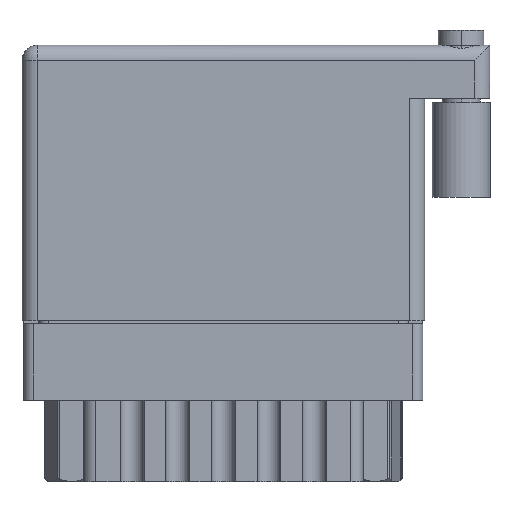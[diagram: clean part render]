
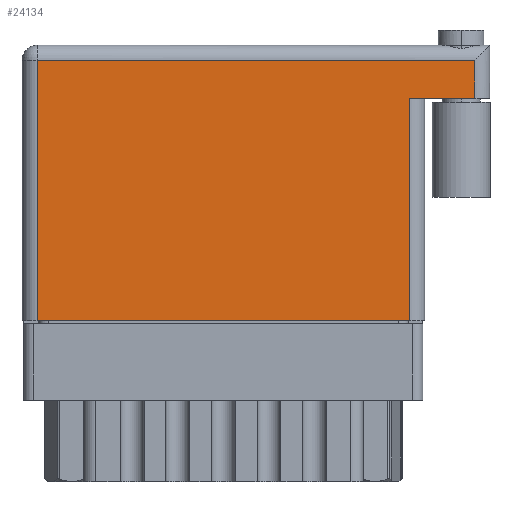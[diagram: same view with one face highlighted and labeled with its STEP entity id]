
A CAD part, front view. The second image highlights one B-rep face of the part: STEP entity #24134.
In plain terms, the highlighted face is planar.
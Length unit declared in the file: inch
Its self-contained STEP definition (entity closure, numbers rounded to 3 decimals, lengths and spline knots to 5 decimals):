
#232 = VERTEX_POINT ( 'NONE', #13580 ) ;
#2009 = VECTOR ( 'NONE', #30860, 39.37008 ) ;
#3985 = ORIENTED_EDGE ( 'NONE', *, *, #11183, .F. ) ;
#5932 = EDGE_CURVE ( 'NONE', #20875, #232, #14091, .T. ) ;
#7931 = DIRECTION ( 'NONE',  ( 0., 1., 0. ) ) ;
#8448 = CARTESIAN_POINT ( 'NONE',  ( 0.05, 0., 0. ) ) ;
#8861 = AXIS2_PLACEMENT_3D ( 'NONE', #38908, #38704, #26793 ) ;
#8960 = LINE ( 'NONE', #15332, #36644 ) ;
#11183 = EDGE_CURVE ( 'NONE', #28005, #23775, #39062, .T. ) ;
#11410 = EDGE_CURVE ( 'NONE', #28005, #20875, #13352, .T. ) ;
#12727 = ORIENTED_EDGE ( 'NONE', *, *, #14842, .T. ) ;
#13352 = LINE ( 'NONE', #16161, #31296 ) ;
#13580 = CARTESIAN_POINT ( 'NONE',  ( 0.05, 0.856, 0. ) ) ;
#14091 = LINE ( 'NONE', #25480, #29832 ) ;
#14234 = DIRECTION ( 'NONE',  ( 0., -1., 0. ) ) ;
#14842 = EDGE_CURVE ( 'NONE', #23801, #23775, #22688, .T. ) ;
#15332 = CARTESIAN_POINT ( 'NONE',  ( 0., 0., 0. ) ) ;
#15533 = DIRECTION ( 'NONE',  ( 1., 0., 0. ) ) ;
#16161 = CARTESIAN_POINT ( 'NONE',  ( 1.489, 0.906, 0. ) ) ;
#16355 = DIRECTION ( 'NONE',  ( 0., 1., 0. ) ) ;
#19970 = EDGE_LOOP ( 'NONE', ( #35298, #12727, #3985, #24122, #21728, #23986 ) ) ;
#20875 = VERTEX_POINT ( 'NONE', #35259 ) ;
#21116 = CARTESIAN_POINT ( 'NONE',  ( 1.275, 0., 0. ) ) ;
#21728 = ORIENTED_EDGE ( 'NONE', *, *, #5932, .T. ) ;
#22688 = LINE ( 'NONE', #35198, #36094 ) ;
#23229 = LINE ( 'NONE', #29376, #23537 ) ;
#23537 = VECTOR ( 'NONE', #14234, 39.37008 ) ;
#23775 = VERTEX_POINT ( 'NONE', #29661 ) ;
#23801 = VERTEX_POINT ( 'NONE', #21116 ) ;
#23986 = ORIENTED_EDGE ( 'NONE', *, *, #24124, .T. ) ;
#24122 = ORIENTED_EDGE ( 'NONE', *, *, #11410, .T. ) ;
#24124 = EDGE_CURVE ( 'NONE', #232, #25932, #23229, .T. ) ;
#24134 = ADVANCED_FACE ( 'NONE', ( #26011 ), #29575, .F. ) ;
#25480 = CARTESIAN_POINT ( 'NONE',  ( 0., 0.856, 0. ) ) ;
#25932 = VERTEX_POINT ( 'NONE', #8448 ) ;
#26011 = FACE_OUTER_BOUND ( 'NONE', #19970, .T. ) ;
#26793 = DIRECTION ( 'NONE',  ( -1., 0., 0. ) ) ;
#28005 = VERTEX_POINT ( 'NONE', #30636 ) ;
#29376 = CARTESIAN_POINT ( 'NONE',  ( 0.05, 0., 0. ) ) ;
#29575 = PLANE ( 'NONE',  #8861 ) ;
#29661 = CARTESIAN_POINT ( 'NONE',  ( 1.275, 0.731, 0. ) ) ;
#29832 = VECTOR ( 'NONE', #37397, 39.37008 ) ;
#30636 = CARTESIAN_POINT ( 'NONE',  ( 1.489, 0.731, 0. ) ) ;
#30860 = DIRECTION ( 'NONE',  ( -1., 0., 0. ) ) ;
#31296 = VECTOR ( 'NONE', #16355, 39.37008 ) ;
#35198 = CARTESIAN_POINT ( 'NONE',  ( 1.275, 0.731, 0. ) ) ;
#35259 = CARTESIAN_POINT ( 'NONE',  ( 1.489, 0.856, 0. ) ) ;
#35298 = ORIENTED_EDGE ( 'NONE', *, *, #37327, .T. ) ;
#36085 = CARTESIAN_POINT ( 'NONE',  ( 1.539, 0.731, 0. ) ) ;
#36094 = VECTOR ( 'NONE', #7931, 39.37008 ) ;
#36644 = VECTOR ( 'NONE', #15533, 39.37008 ) ;
#37327 = EDGE_CURVE ( 'NONE', #25932, #23801, #8960, .T. ) ;
#37397 = DIRECTION ( 'NONE',  ( -1., 0., 0. ) ) ;
#38704 = DIRECTION ( 'NONE',  ( 0., 0., -1. ) ) ;
#38908 = CARTESIAN_POINT ( 'NONE',  ( 0., 0.906, 0. ) ) ;
#39062 = LINE ( 'NONE', #36085, #2009 ) ;
